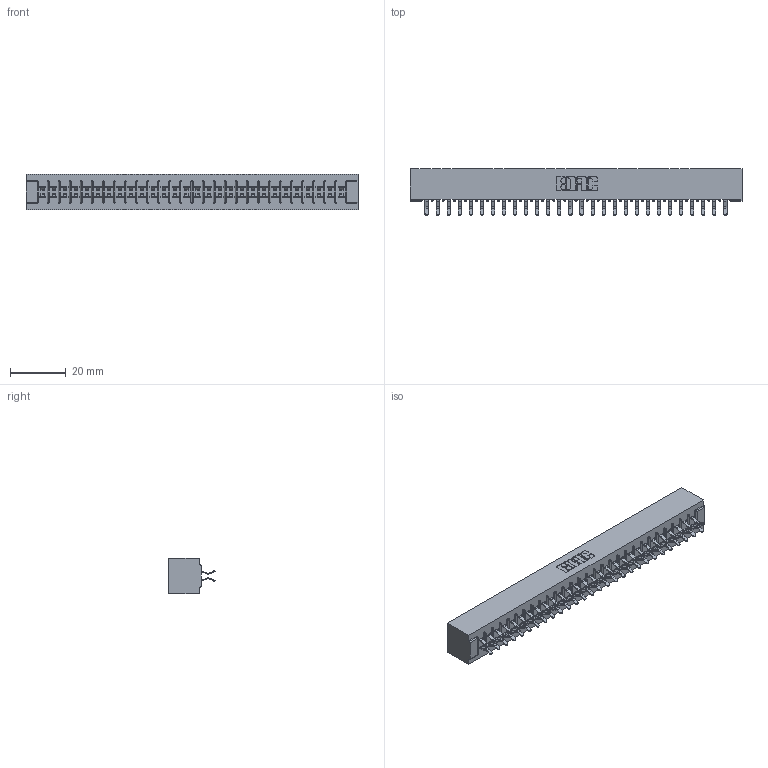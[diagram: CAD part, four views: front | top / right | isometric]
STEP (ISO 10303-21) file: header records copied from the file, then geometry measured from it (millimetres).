
FILE_DESCRIPTION (( 'STEP AP203' ), '1' );
FILE_NAME ('305-056-556-201.STEP', '2019-09-09T23:58:32', ( '' ), ( '' ), 'SwSTEP 2.0', 'SolidWorks 2016', '' );
FILE_SCHEMA (( 'CONFIG_CONTROL_DESIGN' ));
Length unit declared in the file: inch
Products named in the file (3): 305 Part_No Mounting; 305-056-556-201; 305-290-001_556
Assembly tree (57 placements, depth 2):
  305-056-556-201
    305 Part_No Mounting
    305-290-001_556  x56
Bounding box: 118.82 x 16.64 x 12.7 mm (x, y, z)
Volume: 12784.4 mm3; surface area: 16375.2 mm2
Topology: 57 solids, 57 shells, 3244 faces, 9336 edges, 6072 vertices
Faces by surface type: plane 1800, cylinder 1332, sphere 112
Entity records: 31965 total; most frequent: CARTESIAN_POINT 5290, ORIENTED_EDGE 5248, DIRECTION 5130, EDGE_CURVE 2624, LINE 2106, VECTOR 2106, VERTEX_POINT 1672, AXIS2_PLACEMENT_3D 1512
